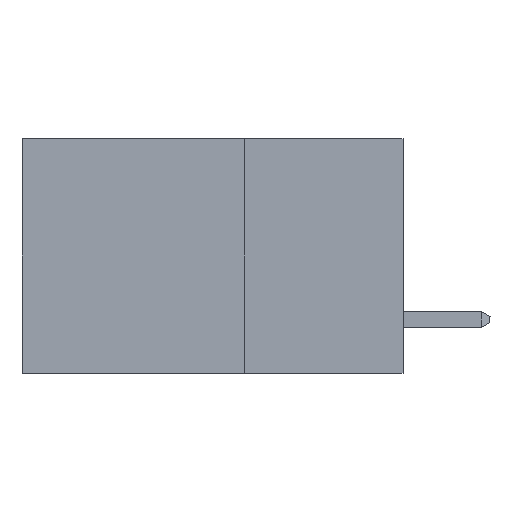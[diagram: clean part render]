
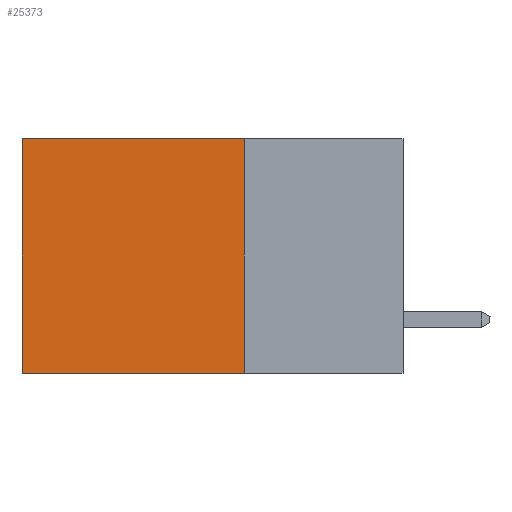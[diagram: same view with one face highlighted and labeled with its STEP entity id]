
A CAD part, left-side view. The second image highlights one B-rep face of the part: STEP entity #25373.
In plain terms, the highlighted planar face has unit normal (-1, 0, 0).
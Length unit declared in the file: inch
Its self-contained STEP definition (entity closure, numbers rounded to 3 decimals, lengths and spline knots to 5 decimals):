
#641 = LINE ( 'NONE', #38113, #20580 ) ;
#1648 = LINE ( 'NONE', #20658, #16961 ) ;
#1836 = VERTEX_POINT ( 'NONE', #16426 ) ;
#1918 = PLANE ( 'NONE',  #29159 ) ;
#2998 = CARTESIAN_POINT ( 'NONE',  ( 0.2875, 0.6, 0. ) ) ;
#5122 = VECTOR ( 'NONE', #25302, 39.37008 ) ;
#5164 = CARTESIAN_POINT ( 'NONE',  ( 0.2875, 0.25, 0. ) ) ;
#5681 = ORIENTED_EDGE ( 'NONE', *, *, #24993, .T. ) ;
#6310 = CARTESIAN_POINT ( 'NONE',  ( 0.2875, 0.25, -0.37 ) ) ;
#7409 = EDGE_CURVE ( 'NONE', #24431, #1836, #641, .T. ) ;
#9241 = DIRECTION ( 'NONE',  ( 0., 0., -1. ) ) ;
#10654 = DIRECTION ( 'NONE',  ( 1., 0., 0. ) ) ;
#12009 = ORIENTED_EDGE ( 'NONE', *, *, #7409, .F. ) ;
#13076 = LINE ( 'NONE', #22346, #5122 ) ;
#14270 = CARTESIAN_POINT ( 'NONE',  ( 0.2875, 0.25, 0. ) ) ;
#16426 = CARTESIAN_POINT ( 'NONE',  ( 0.2875, 0.6, -0.37 ) ) ;
#16961 = VECTOR ( 'NONE', #23371, 39.37008 ) ;
#19549 = VERTEX_POINT ( 'NONE', #34458 ) ;
#20580 = VECTOR ( 'NONE', #32156, 39.37008 ) ;
#20658 = CARTESIAN_POINT ( 'NONE',  ( 0.2875, 0.25, 0. ) ) ;
#22346 = CARTESIAN_POINT ( 'NONE',  ( 0.2875, 0.25, 0. ) ) ;
#23371 = DIRECTION ( 'NONE',  ( 0., 1., 0. ) ) ;
#24431 = VERTEX_POINT ( 'NONE', #6310 ) ;
#24715 = FACE_OUTER_BOUND ( 'NONE', #32620, .T. ) ;
#24993 = EDGE_CURVE ( 'NONE', #19549, #1836, #36339, .T. ) ;
#25302 = DIRECTION ( 'NONE',  ( 0., 0., -1. ) ) ;
#25373 = ADVANCED_FACE ( 'NONE', ( #24715 ), #1918, .F. ) ;
#25519 = VERTEX_POINT ( 'NONE', #14270 ) ;
#25883 = DIRECTION ( 'NONE',  ( 0., 0., -1. ) ) ;
#29159 = AXIS2_PLACEMENT_3D ( 'NONE', #5164, #10654, #25883 ) ;
#32156 = DIRECTION ( 'NONE',  ( 0., 1., 0. ) ) ;
#32620 = EDGE_LOOP ( 'NONE', ( #5681, #12009, #37927, #37159 ) ) ;
#33276 = EDGE_CURVE ( 'NONE', #25519, #24431, #13076, .T. ) ;
#34458 = CARTESIAN_POINT ( 'NONE',  ( 0.2875, 0.6, 0. ) ) ;
#36339 = LINE ( 'NONE', #2998, #37747 ) ;
#36777 = EDGE_CURVE ( 'NONE', #25519, #19549, #1648, .T. ) ;
#37159 = ORIENTED_EDGE ( 'NONE', *, *, #36777, .T. ) ;
#37747 = VECTOR ( 'NONE', #9241, 39.37008 ) ;
#37927 = ORIENTED_EDGE ( 'NONE', *, *, #33276, .F. ) ;
#38113 = CARTESIAN_POINT ( 'NONE',  ( 0.2875, 0.25, -0.37 ) ) ;
